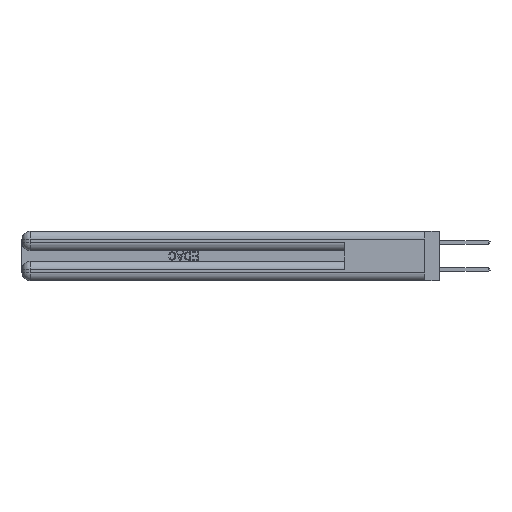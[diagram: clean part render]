
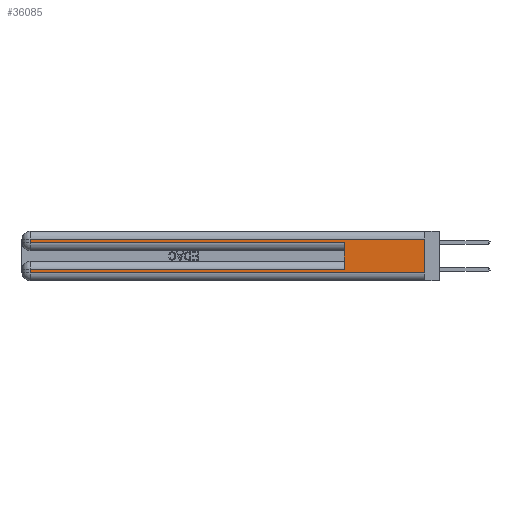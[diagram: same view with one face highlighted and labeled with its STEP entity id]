
A CAD part, left-side view. The second image highlights one B-rep face of the part: STEP entity #36085.
In plain terms, the highlighted planar face has unit normal (-1, 0, 0).
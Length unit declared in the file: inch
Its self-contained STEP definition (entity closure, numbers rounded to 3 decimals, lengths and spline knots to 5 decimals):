
#441 = DIRECTION ( 'NONE',  ( 0., 1., 0. ) ) ;
#999 = CARTESIAN_POINT ( 'NONE',  ( 0., 2.94, 0.37 ) ) ;
#1161 = CARTESIAN_POINT ( 'NONE',  ( 0., 0., 0.06 ) ) ;
#1234 = AXIS2_PLACEMENT_3D ( 'NONE', #17174, #1546, #29342 ) ;
#1546 = DIRECTION ( 'NONE',  ( 1., 0., 0. ) ) ;
#1634 = ORIENTED_EDGE ( 'NONE', *, *, #39565, .T. ) ;
#1795 = LINE ( 'NONE', #1161, #14419 ) ;
#1888 = CARTESIAN_POINT ( 'NONE',  ( 0., 2.94, 0.37 ) ) ;
#2076 = LINE ( 'NONE', #4091, #34563 ) ;
#2343 = VERTEX_POINT ( 'NONE', #14049 ) ;
#2865 = EDGE_CURVE ( 'NONE', #2343, #40189, #34797, .T. ) ;
#3893 = CARTESIAN_POINT ( 'NONE',  ( 0., 0., 0.31 ) ) ;
#4091 = CARTESIAN_POINT ( 'NONE',  ( 0., 0., 0.37 ) ) ;
#4453 = VECTOR ( 'NONE', #441, 39.37008 ) ;
#4837 = VECTOR ( 'NONE', #30436, 39.37008 ) ;
#5384 = CARTESIAN_POINT ( 'NONE',  ( 0., 2.94, 0.06 ) ) ;
#5691 = VERTEX_POINT ( 'NONE', #5384 ) ;
#9264 = VERTEX_POINT ( 'NONE', #37298 ) ;
#9709 = ORIENTED_EDGE ( 'NONE', *, *, #10714, .T. ) ;
#10714 = EDGE_CURVE ( 'NONE', #5691, #30846, #1795, .T. ) ;
#12279 = ORIENTED_EDGE ( 'NONE', *, *, #14664, .T. ) ;
#12491 = EDGE_CURVE ( 'NONE', #36636, #5691, #22063, .T. ) ;
#12765 = ORIENTED_EDGE ( 'NONE', *, *, #35887, .T. ) ;
#13222 = PLANE ( 'NONE',  #1234 ) ;
#13801 = VECTOR ( 'NONE', #23609, 39.37008 ) ;
#14049 = CARTESIAN_POINT ( 'NONE',  ( 0., 2.94, 0.285 ) ) ;
#14419 = VECTOR ( 'NONE', #28852, 39.37008 ) ;
#14664 = EDGE_CURVE ( 'NONE', #33183, #40053, #24813, .T. ) ;
#15233 = VECTOR ( 'NONE', #37955, 39.37008 ) ;
#15955 = CARTESIAN_POINT ( 'NONE',  ( 0., 0., 0.31 ) ) ;
#16406 = ORIENTED_EDGE ( 'NONE', *, *, #12491, .T. ) ;
#17174 = CARTESIAN_POINT ( 'NONE',  ( 0., 0., 0.37 ) ) ;
#18364 = CARTESIAN_POINT ( 'NONE',  ( 0., 0., 0.085 ) ) ;
#18505 = CARTESIAN_POINT ( 'NONE',  ( 0., 2.94, 0.31 ) ) ;
#19125 = LINE ( 'NONE', #999, #15233 ) ;
#22063 = LINE ( 'NONE', #1888, #13801 ) ;
#22242 = EDGE_CURVE ( 'NONE', #9264, #40189, #22596, .T. ) ;
#22283 = CARTESIAN_POINT ( 'NONE',  ( 0., 2.94, 0.085 ) ) ;
#22596 = LINE ( 'NONE', #39613, #30404 ) ;
#23609 = DIRECTION ( 'NONE',  ( 0., 0., -1. ) ) ;
#24150 = DIRECTION ( 'NONE',  ( 0., 0., 1. ) ) ;
#24153 = VECTOR ( 'NONE', #32017, 39.37008 ) ;
#24257 = LINE ( 'NONE', #18364, #4837 ) ;
#24473 = ORIENTED_EDGE ( 'NONE', *, *, #22242, .F. ) ;
#24547 = EDGE_CURVE ( 'NONE', #33183, #30846, #2076, .T. ) ;
#24813 = LINE ( 'NONE', #15955, #4453 ) ;
#24877 = CARTESIAN_POINT ( 'NONE',  ( 0., 0.6, 0.285 ) ) ;
#25154 = FACE_OUTER_BOUND ( 'NONE', #29850, .T. ) ;
#28375 = CARTESIAN_POINT ( 'NONE',  ( 0., 0., 0.06 ) ) ;
#28852 = DIRECTION ( 'NONE',  ( 0., -1., 0. ) ) ;
#29171 = ORIENTED_EDGE ( 'NONE', *, *, #2865, .T. ) ;
#29342 = DIRECTION ( 'NONE',  ( 0., 0., -1. ) ) ;
#29850 = EDGE_LOOP ( 'NONE', ( #30594, #12279, #1634, #29171, #24473, #12765, #16406, #9709 ) ) ;
#30404 = VECTOR ( 'NONE', #24150, 39.37008 ) ;
#30436 = DIRECTION ( 'NONE',  ( 0., 1., 0. ) ) ;
#30594 = ORIENTED_EDGE ( 'NONE', *, *, #24547, .F. ) ;
#30692 = CARTESIAN_POINT ( 'NONE',  ( 0., 0., 0.285 ) ) ;
#30846 = VERTEX_POINT ( 'NONE', #28375 ) ;
#32017 = DIRECTION ( 'NONE',  ( 0., -1., 0. ) ) ;
#33183 = VERTEX_POINT ( 'NONE', #3893 ) ;
#34563 = VECTOR ( 'NONE', #34619, 39.37008 ) ;
#34619 = DIRECTION ( 'NONE',  ( 0., 0., -1. ) ) ;
#34797 = LINE ( 'NONE', #30692, #24153 ) ;
#35887 = EDGE_CURVE ( 'NONE', #9264, #36636, #24257, .T. ) ;
#36085 = ADVANCED_FACE ( 'NONE', ( #25154 ), #13222, .F. ) ;
#36636 = VERTEX_POINT ( 'NONE', #22283 ) ;
#37298 = CARTESIAN_POINT ( 'NONE',  ( 0., 0.6, 0.085 ) ) ;
#37955 = DIRECTION ( 'NONE',  ( 0., 0., -1. ) ) ;
#39565 = EDGE_CURVE ( 'NONE', #40053, #2343, #19125, .T. ) ;
#39613 = CARTESIAN_POINT ( 'NONE',  ( 0., 0.6, 0.145 ) ) ;
#40053 = VERTEX_POINT ( 'NONE', #18505 ) ;
#40189 = VERTEX_POINT ( 'NONE', #24877 ) ;
